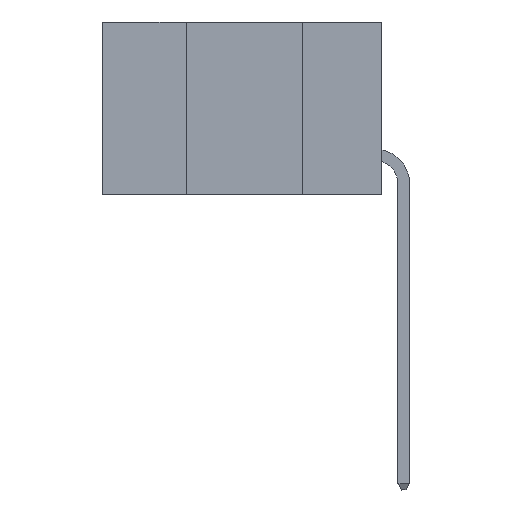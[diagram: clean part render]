
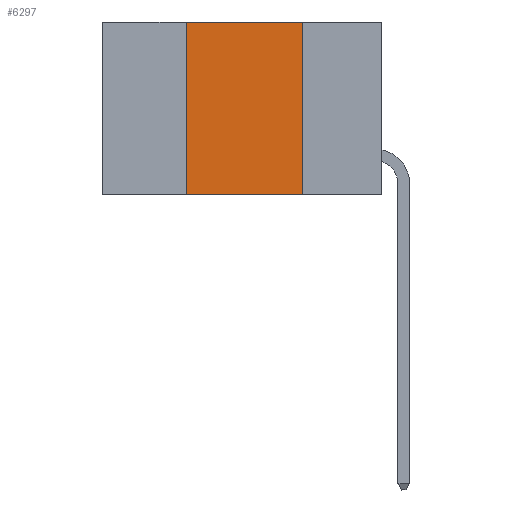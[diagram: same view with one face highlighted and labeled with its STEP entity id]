
A CAD part, left-side view. The second image highlights one B-rep face of the part: STEP entity #6297.
In plain terms, the highlighted planar face has unit normal (-1, 0, 0).
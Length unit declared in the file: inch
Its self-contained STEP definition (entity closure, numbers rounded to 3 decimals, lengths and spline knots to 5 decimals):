
#2517 = ORIENTED_EDGE ( 'NONE', *, *, #27251, .F. ) ;
#3313 = LINE ( 'NONE', #34452, #9563 ) ;
#4645 = CARTESIAN_POINT ( 'NONE',  ( 0., 0.42, 0. ) ) ;
#6017 = ORIENTED_EDGE ( 'NONE', *, *, #34674, .T. ) ;
#6297 = ADVANCED_FACE ( 'NONE', ( #12903 ), #19975, .F. ) ;
#7156 = DIRECTION ( 'NONE',  ( 0., 0., -1. ) ) ;
#7988 = DIRECTION ( 'NONE',  ( 1., 0., 0. ) ) ;
#8462 = EDGE_CURVE ( 'NONE', #21020, #14703, #33890, .T. ) ;
#9563 = VECTOR ( 'NONE', #31474, 39.37008 ) ;
#11527 = VECTOR ( 'NONE', #33370, 39.37008 ) ;
#12903 = FACE_OUTER_BOUND ( 'NONE', #35242, .T. ) ;
#13603 = CARTESIAN_POINT ( 'NONE',  ( 0., 0.6, 0. ) ) ;
#13747 = ORIENTED_EDGE ( 'NONE', *, *, #17578, .F. ) ;
#14703 = VERTEX_POINT ( 'NONE', #14774 ) ;
#14774 = CARTESIAN_POINT ( 'NONE',  ( 0., 0.42, 0. ) ) ;
#16983 = DIRECTION ( 'NONE',  ( 0., 0., -1. ) ) ;
#17578 = EDGE_CURVE ( 'NONE', #36303, #18802, #28213, .T. ) ;
#18260 = LINE ( 'NONE', #33106, #11527 ) ;
#18802 = VERTEX_POINT ( 'NONE', #18913 ) ;
#18913 = CARTESIAN_POINT ( 'NONE',  ( 0., 0.17, -0.37 ) ) ;
#19666 = CARTESIAN_POINT ( 'NONE',  ( 0., 0.17, 0. ) ) ;
#19975 = PLANE ( 'NONE',  #31411 ) ;
#21020 = VERTEX_POINT ( 'NONE', #23682 ) ;
#23682 = CARTESIAN_POINT ( 'NONE',  ( 0., 0.42, -0.37 ) ) ;
#24383 = VECTOR ( 'NONE', #7156, 39.37008 ) ;
#27251 = EDGE_CURVE ( 'NONE', #14703, #36303, #3313, .T. ) ;
#28213 = LINE ( 'NONE', #19666, #24383 ) ;
#31411 = AXIS2_PLACEMENT_3D ( 'NONE', #13603, #7988, #16983 ) ;
#31474 = DIRECTION ( 'NONE',  ( 0., -1., 0. ) ) ;
#33106 = CARTESIAN_POINT ( 'NONE',  ( 0., 0.6, -0.37 ) ) ;
#33370 = DIRECTION ( 'NONE',  ( 0., -1., 0. ) ) ;
#33890 = LINE ( 'NONE', #4645, #35271 ) ;
#34452 = CARTESIAN_POINT ( 'NONE',  ( 0., 0.6, 0. ) ) ;
#34674 = EDGE_CURVE ( 'NONE', #21020, #18802, #18260, .T. ) ;
#35242 = EDGE_LOOP ( 'NONE', ( #13747, #2517, #39781, #6017 ) ) ;
#35271 = VECTOR ( 'NONE', #38843, 39.37008 ) ;
#36303 = VERTEX_POINT ( 'NONE', #36615 ) ;
#36615 = CARTESIAN_POINT ( 'NONE',  ( 0., 0.17, 0. ) ) ;
#38843 = DIRECTION ( 'NONE',  ( 0., 0., 1. ) ) ;
#39781 = ORIENTED_EDGE ( 'NONE', *, *, #8462, .F. ) ;
